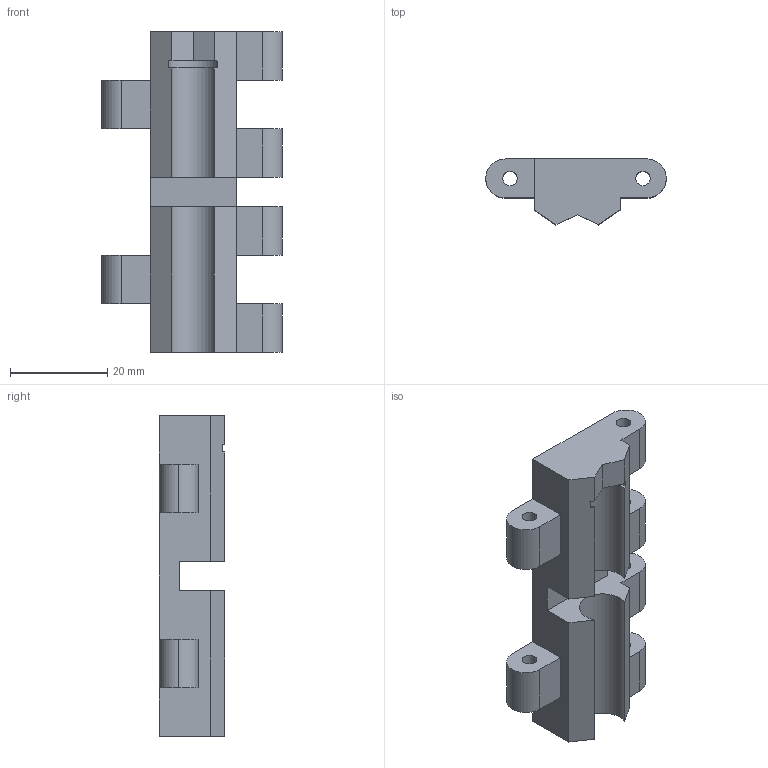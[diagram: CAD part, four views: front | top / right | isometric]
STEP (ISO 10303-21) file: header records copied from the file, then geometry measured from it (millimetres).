
FILE_DESCRIPTION (( 'STEP AP214' ), '1' );
FILE_NAME ('Belt 2.0 5.56.STEP', '2025-05-18T10:37:40', ( '' ), ( '' ), 'SwSTEP 2.0', 'SolidWorks 2024', '' );
FILE_SCHEMA (( 'AUTOMOTIVE_DESIGN' ));
Length unit declared in the file: millimetre
Products named in the file (1): Belt 2.0 5.56
Bounding box: 37.1 x 13.5 x 66 mm (x, y, z)
Volume: 14677.6 mm3; surface area: 7235.1 mm2
Topology: 1 solids, 1 shells, 65 faces, 189 edges, 126 vertices
Faces by surface type: cylinder 33, plane 32
Entity records: 2216 total; most frequent: DIRECTION 387, CARTESIAN_POINT 381, ORIENTED_EDGE 378, EDGE_CURVE 189, AXIS2_PLACEMENT_3D 132, VERTEX_POINT 126, LINE 123, VECTOR 123
